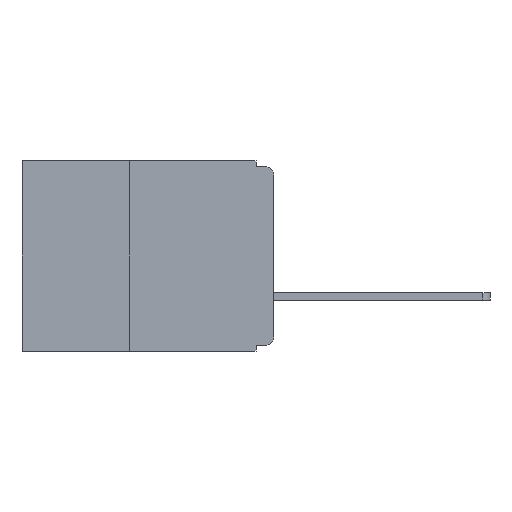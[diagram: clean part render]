
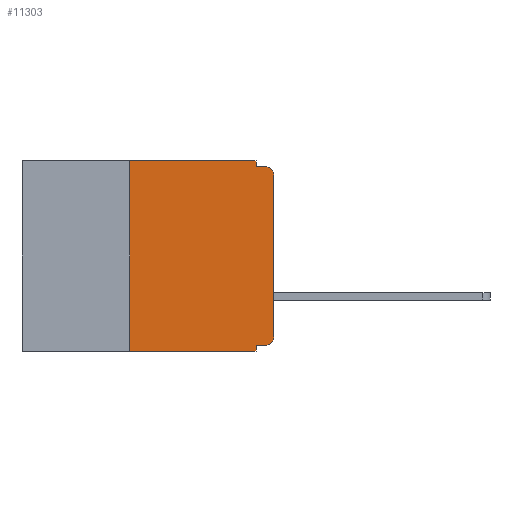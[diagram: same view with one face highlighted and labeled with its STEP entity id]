
A CAD part, left-side view. The second image highlights one B-rep face of the part: STEP entity #11303.
In plain terms, the highlighted planar face has unit normal (-1, 0, 0).
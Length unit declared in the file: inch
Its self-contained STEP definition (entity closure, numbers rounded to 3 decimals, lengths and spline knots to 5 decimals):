
#267 = CARTESIAN_POINT ( 'NONE',  ( 0., 0.25, 0. ) ) ;
#610 = CARTESIAN_POINT ( 'NONE',  ( 0., 0., -0.025 ) ) ;
#888 = ORIENTED_EDGE ( 'NONE', *, *, #7637, .T. ) ;
#902 = CARTESIAN_POINT ( 'NONE',  ( 0., 0.25, -0.33 ) ) ;
#1235 = DIRECTION ( 'NONE',  ( 1., 0., 0. ) ) ;
#1694 = LINE ( 'NONE', #5685, #10851 ) ;
#1725 = ORIENTED_EDGE ( 'NONE', *, *, #7346, .T. ) ;
#1806 = DIRECTION ( 'NONE',  ( 0., 0., -1. ) ) ;
#1874 = VERTEX_POINT ( 'NONE', #11593 ) ;
#1942 = DIRECTION ( 'NONE',  ( -1., 0., 0. ) ) ;
#1950 = CARTESIAN_POINT ( 'NONE',  ( 0., 0.015, -0.305 ) ) ;
#2117 = VECTOR ( 'NONE', #7569, 39.37008 ) ;
#2380 = AXIS2_PLACEMENT_3D ( 'NONE', #11880, #1235, #8179 ) ;
#2452 = EDGE_CURVE ( 'NONE', #7726, #6592, #7751, .T. ) ;
#2589 = DIRECTION ( 'NONE',  ( 0., 0., -1. ) ) ;
#2696 = DIRECTION ( 'NONE',  ( -1., 0., 0. ) ) ;
#2773 = CARTESIAN_POINT ( 'NONE',  ( 0., 0.015, -0.025 ) ) ;
#3142 = DIRECTION ( 'NONE',  ( 0., 0., -1. ) ) ;
#3227 = CARTESIAN_POINT ( 'NONE',  ( 0., 0.031, -0.33 ) ) ;
#3282 = ORIENTED_EDGE ( 'NONE', *, *, #8938, .F. ) ;
#3438 = CARTESIAN_POINT ( 'NONE',  ( 0., 0., -0.305 ) ) ;
#3859 = LINE ( 'NONE', #3227, #10653 ) ;
#4113 = VERTEX_POINT ( 'NONE', #10151 ) ;
#4445 = CARTESIAN_POINT ( 'NONE',  ( 0., 0.031, 0. ) ) ;
#4487 = CARTESIAN_POINT ( 'NONE',  ( 0., 0.031, -0.01 ) ) ;
#4496 = VECTOR ( 'NONE', #6625, 39.37008 ) ;
#4703 = ORIENTED_EDGE ( 'NONE', *, *, #7575, .F. ) ;
#4756 = CARTESIAN_POINT ( 'NONE',  ( 0., 0.031, -0.32 ) ) ;
#4850 = ORIENTED_EDGE ( 'NONE', *, *, #8885, .F. ) ;
#4951 = DIRECTION ( 'NONE',  ( 0., -1., 0. ) ) ;
#5313 = DIRECTION ( 'NONE',  ( 0., 1., 0. ) ) ;
#5315 = VERTEX_POINT ( 'NONE', #4487 ) ;
#5372 = CARTESIAN_POINT ( 'NONE',  ( 0., 0., -0.32 ) ) ;
#5685 = CARTESIAN_POINT ( 'NONE',  ( 0., 0.437, -0.33 ) ) ;
#5792 = CARTESIAN_POINT ( 'NONE',  ( 0., 0.25, -0.33 ) ) ;
#5954 = CIRCLE ( 'NONE', #6280, 0.015 ) ;
#6046 = CIRCLE ( 'NONE', #6109, 0.015 ) ;
#6050 = FACE_OUTER_BOUND ( 'NONE', #8627, .T. ) ;
#6109 = AXIS2_PLACEMENT_3D ( 'NONE', #2773, #2696, #2589 ) ;
#6228 = ORIENTED_EDGE ( 'NONE', *, *, #7480, .F. ) ;
#6280 = AXIS2_PLACEMENT_3D ( 'NONE', #1950, #1942, #1806 ) ;
#6438 = VECTOR ( 'NONE', #5313, 39.37008 ) ;
#6467 = LINE ( 'NONE', #5372, #6438 ) ;
#6565 = VERTEX_POINT ( 'NONE', #4756 ) ;
#6592 = VERTEX_POINT ( 'NONE', #4445 ) ;
#6625 = DIRECTION ( 'NONE',  ( 0., 0., 1. ) ) ;
#6946 = VECTOR ( 'NONE', #8158, 39.37008 ) ;
#7058 = VERTEX_POINT ( 'NONE', #610 ) ;
#7078 = CARTESIAN_POINT ( 'NONE',  ( 0., 0.031, 0. ) ) ;
#7346 = EDGE_CURVE ( 'NONE', #7647, #7058, #8634, .T. ) ;
#7406 = LINE ( 'NONE', #8796, #6946 ) ;
#7480 = EDGE_CURVE ( 'NONE', #5315, #10984, #7406, .T. ) ;
#7569 = DIRECTION ( 'NONE',  ( 0., 0., -1. ) ) ;
#7575 = EDGE_CURVE ( 'NONE', #4113, #6565, #6467, .T. ) ;
#7623 = EDGE_CURVE ( 'NONE', #7058, #10984, #6046, .T. ) ;
#7637 = EDGE_CURVE ( 'NONE', #4113, #7647, #5954, .T. ) ;
#7647 = VERTEX_POINT ( 'NONE', #3438 ) ;
#7684 = VECTOR ( 'NONE', #7864, 39.37008 ) ;
#7706 = CARTESIAN_POINT ( 'NONE',  ( 0., 0.015, -0.01 ) ) ;
#7726 = VERTEX_POINT ( 'NONE', #267 ) ;
#7751 = LINE ( 'NONE', #11501, #7684 ) ;
#7864 = DIRECTION ( 'NONE',  ( 0., -1., 0. ) ) ;
#8106 = ORIENTED_EDGE ( 'NONE', *, *, #2452, .F. ) ;
#8158 = DIRECTION ( 'NONE',  ( 0., -1., 0. ) ) ;
#8179 = DIRECTION ( 'NONE',  ( 0., 0., -1. ) ) ;
#8627 = EDGE_LOOP ( 'NONE', ( #1725, #9921, #6228, #8664, #8106, #4850, #9003, #3282, #4703, #888 ) ) ;
#8634 = LINE ( 'NONE', #11187, #8772 ) ;
#8664 = ORIENTED_EDGE ( 'NONE', *, *, #8853, .F. ) ;
#8772 = VECTOR ( 'NONE', #11330, 39.37008 ) ;
#8796 = CARTESIAN_POINT ( 'NONE',  ( 0., 0., -0.01 ) ) ;
#8853 = EDGE_CURVE ( 'NONE', #6592, #5315, #11470, .T. ) ;
#8885 = EDGE_CURVE ( 'NONE', #10036, #7726, #9588, .T. ) ;
#8910 = EDGE_CURVE ( 'NONE', #10036, #1874, #1694, .T. ) ;
#8938 = EDGE_CURVE ( 'NONE', #6565, #1874, #3859, .T. ) ;
#8984 = PLANE ( 'NONE',  #2380 ) ;
#9003 = ORIENTED_EDGE ( 'NONE', *, *, #8910, .T. ) ;
#9588 = LINE ( 'NONE', #5792, #4496 ) ;
#9921 = ORIENTED_EDGE ( 'NONE', *, *, #7623, .T. ) ;
#10036 = VERTEX_POINT ( 'NONE', #902 ) ;
#10151 = CARTESIAN_POINT ( 'NONE',  ( 0., 0.015, -0.32 ) ) ;
#10653 = VECTOR ( 'NONE', #3142, 39.37008 ) ;
#10851 = VECTOR ( 'NONE', #4951, 39.37008 ) ;
#10984 = VERTEX_POINT ( 'NONE', #7706 ) ;
#11187 = CARTESIAN_POINT ( 'NONE',  ( 0., 0., 0. ) ) ;
#11303 = ADVANCED_FACE ( 'NONE', ( #6050 ), #8984, .F. ) ;
#11330 = DIRECTION ( 'NONE',  ( 0., 0., 1. ) ) ;
#11470 = LINE ( 'NONE', #7078, #2117 ) ;
#11501 = CARTESIAN_POINT ( 'NONE',  ( 0., 0.437, 0. ) ) ;
#11593 = CARTESIAN_POINT ( 'NONE',  ( 0., 0.031, -0.33 ) ) ;
#11880 = CARTESIAN_POINT ( 'NONE',  ( 0., 0.437, 0. ) ) ;
